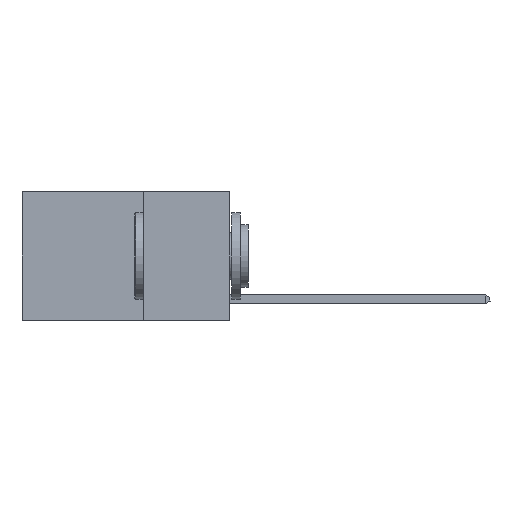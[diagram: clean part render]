
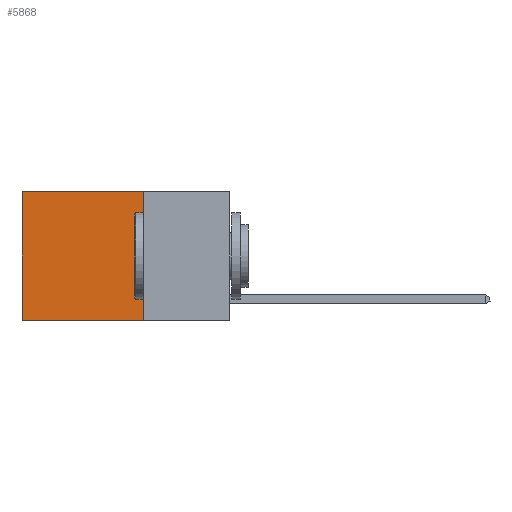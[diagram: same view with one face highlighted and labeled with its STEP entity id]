
A CAD part, left-side view. The second image highlights one B-rep face of the part: STEP entity #5868.
In plain terms, the highlighted planar face has unit normal (-1, 0, 0).
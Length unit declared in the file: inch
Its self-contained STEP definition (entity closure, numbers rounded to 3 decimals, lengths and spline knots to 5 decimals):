
#1237 = ORIENTED_EDGE ( 'NONE', *, *, #18348, .F. ) ;
#3163 = CARTESIAN_POINT ( 'NONE',  ( 0.2625, 0.25, 0. ) ) ;
#4025 = EDGE_LOOP ( 'NONE', ( #11392, #1237, #4789, #17537 ) ) ;
#4367 = VERTEX_POINT ( 'NONE', #15626 ) ;
#4571 = CARTESIAN_POINT ( 'NONE',  ( 0.2625, 0.6, 0. ) ) ;
#4789 = ORIENTED_EDGE ( 'NONE', *, *, #18455, .F. ) ;
#5113 = DIRECTION ( 'NONE',  ( 0., 1., 0. ) ) ;
#5868 = ADVANCED_FACE ( 'NONE', ( #17392 ), #20658, .F. ) ;
#6152 = CARTESIAN_POINT ( 'NONE',  ( 0.2625, 0.25, 0. ) ) ;
#6730 = VERTEX_POINT ( 'NONE', #7524 ) ;
#7412 = LINE ( 'NONE', #20174, #11649 ) ;
#7524 = CARTESIAN_POINT ( 'NONE',  ( 0.2625, 0.25, 0. ) ) ;
#7911 = DIRECTION ( 'NONE',  ( 0., 0., -1. ) ) ;
#10577 = VECTOR ( 'NONE', #7911, 39.37008 ) ;
#11267 = DIRECTION ( 'NONE',  ( 0., 0., -1. ) ) ;
#11392 = ORIENTED_EDGE ( 'NONE', *, *, #15578, .T. ) ;
#11649 = VECTOR ( 'NONE', #13844, 39.37008 ) ;
#12241 = VECTOR ( 'NONE', #20809, 39.37008 ) ;
#12668 = LINE ( 'NONE', #19203, #10577 ) ;
#13106 = EDGE_CURVE ( 'NONE', #6730, #13814, #18624, .T. ) ;
#13814 = VERTEX_POINT ( 'NONE', #4571 ) ;
#13844 = DIRECTION ( 'NONE',  ( 0., 0., -1. ) ) ;
#14914 = LINE ( 'NONE', #16605, #18376 ) ;
#15578 = EDGE_CURVE ( 'NONE', #13814, #4367, #12668, .T. ) ;
#15626 = CARTESIAN_POINT ( 'NONE',  ( 0.2625, 0.6, -0.37 ) ) ;
#15921 = DIRECTION ( 'NONE',  ( 1., 0., 0. ) ) ;
#16305 = CARTESIAN_POINT ( 'NONE',  ( 0.2625, 0.25, -0.37 ) ) ;
#16605 = CARTESIAN_POINT ( 'NONE',  ( 0.2625, 0.25, -0.37 ) ) ;
#17392 = FACE_OUTER_BOUND ( 'NONE', #4025, .T. ) ;
#17537 = ORIENTED_EDGE ( 'NONE', *, *, #13106, .T. ) ;
#17803 = AXIS2_PLACEMENT_3D ( 'NONE', #3163, #15921, #11267 ) ;
#18348 = EDGE_CURVE ( 'NONE', #20695, #4367, #14914, .T. ) ;
#18376 = VECTOR ( 'NONE', #5113, 39.37008 ) ;
#18455 = EDGE_CURVE ( 'NONE', #6730, #20695, #7412, .T. ) ;
#18624 = LINE ( 'NONE', #6152, #12241 ) ;
#19203 = CARTESIAN_POINT ( 'NONE',  ( 0.2625, 0.6, 0. ) ) ;
#20174 = CARTESIAN_POINT ( 'NONE',  ( 0.2625, 0.25, 0. ) ) ;
#20658 = PLANE ( 'NONE',  #17803 ) ;
#20695 = VERTEX_POINT ( 'NONE', #16305 ) ;
#20809 = DIRECTION ( 'NONE',  ( 0., 1., 0. ) ) ;
